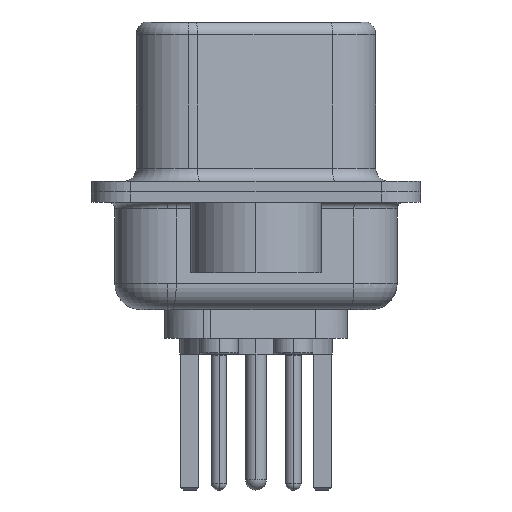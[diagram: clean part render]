
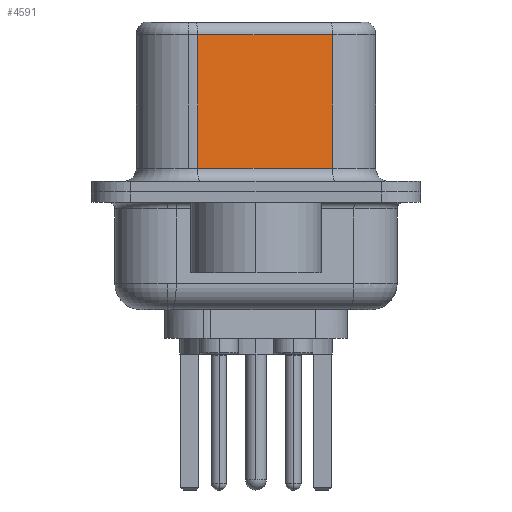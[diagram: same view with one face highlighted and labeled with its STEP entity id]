
A CAD part, left-side view. The second image highlights one B-rep face of the part: STEP entity #4591.
In plain terms, the highlighted planar face has unit normal (-0.985, -0.174, 0).
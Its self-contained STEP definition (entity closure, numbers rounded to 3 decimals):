
#333 = VERTEX_POINT ( 'NONE', #8514 ) ;
#508 = CARTESIAN_POINT ( 'NONE',  ( 3.67, 2.233, 6.02 ) ) ;
#1280 = CARTESIAN_POINT ( 'NONE',  ( 3.67, 2.233, 0.9 ) ) ;
#1331 = VECTOR ( 'NONE', #12850, 1000. ) ;
#1789 = LINE ( 'NONE', #12051, #1331 ) ;
#2780 = EDGE_CURVE ( 'NONE', #6882, #7471, #1789, .T. ) ;
#2936 = FACE_OUTER_BOUND ( 'NONE', #13933, .T. ) ;
#3665 = VECTOR ( 'NONE', #9390, 1000. ) ;
#4125 = AXIS2_PLACEMENT_3D ( 'NONE', #13291, #16333, #17419 ) ;
#4175 = EDGE_CURVE ( 'NONE', #10941, #333, #11694, .T. ) ;
#4586 = DIRECTION ( 'NONE',  ( 0.174, -0.985, 0. ) ) ;
#4591 = ADVANCED_FACE ( 'NONE', ( #2936 ), #13917, .F. ) ;
#4909 = LINE ( 'NONE', #7719, #12515 ) ;
#5912 = VECTOR ( 'NONE', #4586, 1000. ) ;
#6210 = CARTESIAN_POINT ( 'NONE',  ( 4.58, -2.927, 6.52 ) ) ;
#6882 = VERTEX_POINT ( 'NONE', #508 ) ;
#7471 = VERTEX_POINT ( 'NONE', #1280 ) ;
#7719 = CARTESIAN_POINT ( 'NONE',  ( 4.58, -2.927, 6.02 ) ) ;
#8188 = EDGE_CURVE ( 'NONE', #7471, #333, #13944, .T. ) ;
#8514 = CARTESIAN_POINT ( 'NONE',  ( 4.58, -2.927, 0.9 ) ) ;
#9390 = DIRECTION ( 'NONE',  ( 0., 0., -1. ) ) ;
#9517 = EDGE_CURVE ( 'NONE', #10941, #6882, #4909, .T. ) ;
#10473 = CARTESIAN_POINT ( 'NONE',  ( 4.58, -2.927, 0.9 ) ) ;
#10722 = CARTESIAN_POINT ( 'NONE',  ( 4.58, -2.927, 6.02 ) ) ;
#10941 = VERTEX_POINT ( 'NONE', #10722 ) ;
#11024 = ORIENTED_EDGE ( 'NONE', *, *, #8188, .T. ) ;
#11694 = LINE ( 'NONE', #6210, #3665 ) ;
#12051 = CARTESIAN_POINT ( 'NONE',  ( 3.67, 2.233, 6.52 ) ) ;
#12515 = VECTOR ( 'NONE', #13696, 1000. ) ;
#12850 = DIRECTION ( 'NONE',  ( 0., 0., -1. ) ) ;
#13291 = CARTESIAN_POINT ( 'NONE',  ( 4.58, -2.927, 6.52 ) ) ;
#13696 = DIRECTION ( 'NONE',  ( -0.174, 0.985, 0. ) ) ;
#13917 = PLANE ( 'NONE',  #4125 ) ;
#13933 = EDGE_LOOP ( 'NONE', ( #16072, #15334, #17637, #11024 ) ) ;
#13944 = LINE ( 'NONE', #10473, #5912 ) ;
#15334 = ORIENTED_EDGE ( 'NONE', *, *, #9517, .T. ) ;
#16072 = ORIENTED_EDGE ( 'NONE', *, *, #4175, .F. ) ;
#16333 = DIRECTION ( 'NONE',  ( 0.985, 0.174, 0. ) ) ;
#17419 = DIRECTION ( 'NONE',  ( -0.174, 0.985, 0. ) ) ;
#17637 = ORIENTED_EDGE ( 'NONE', *, *, #2780, .T. ) ;
